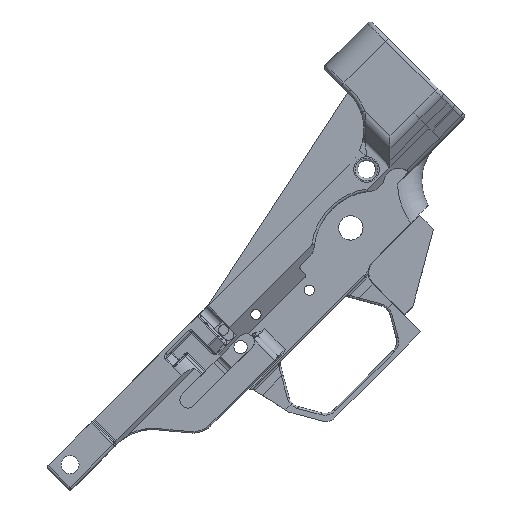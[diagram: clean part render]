
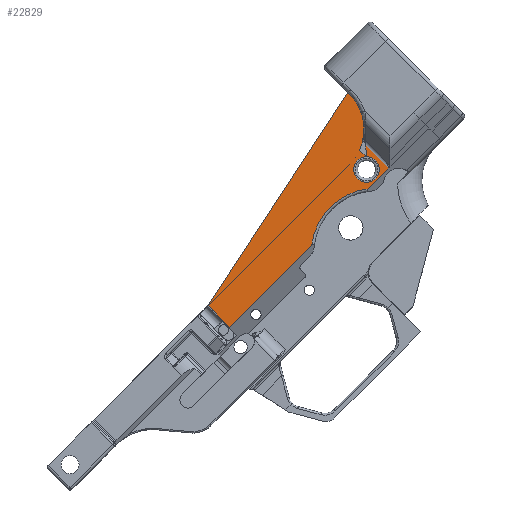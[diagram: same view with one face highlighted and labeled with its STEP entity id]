
A CAD part, front view. The second image highlights one B-rep face of the part: STEP entity #22829.
In plain terms, the highlighted planar face has unit normal (0, -1, 0).
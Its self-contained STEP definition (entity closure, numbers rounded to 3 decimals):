
#5562=CARTESIAN_POINT('',(-25.441,-18.567,22.339));
#5563=VERTEX_POINT('',#5562);
#5571=CARTESIAN_POINT('',(29.722,-18.567,77.502));
#5572=VERTEX_POINT('',#5571);
#5573=CARTESIAN_POINT('',(29.722,-18.567,77.502));
#5574=DIRECTION('',(-0.707,0.0,-0.707));
#5575=VECTOR('',#5574,78.013);
#5576=LINE('',#5573,#5575);
#5577=EDGE_CURVE('',#5572,#5563,#5576,.T.);
#9678=CARTESIAN_POINT('',(45.024,-18.567,76.019));
#9679=VERTEX_POINT('',#9678);
#9686=CARTESIAN_POINT('',(36.922,-18.567,67.916));
#9687=VERTEX_POINT('',#9686);
#9688=CARTESIAN_POINT('',(45.024,-18.567,76.019));
#9689=DIRECTION('',(-0.707,0.,-0.707));
#9690=VECTOR('',#9689,11.459);
#9691=LINE('',#9688,#9690);
#9692=EDGE_CURVE('',#9679,#9687,#9691,.T.);
#10764=CARTESIAN_POINT('',(41.289,-18.567,75.425));
#10765=VERTEX_POINT('',#10764);
#10766=CARTESIAN_POINT('',(36.289,-18.567,75.425));
#10767=DIRECTION('',(0.0,-1.0,0.0));
#10768=DIRECTION('',(1.0,0.0,0.0));
#10769=AXIS2_PLACEMENT_3D('',#10766,#10767,#10768);
#10770=CIRCLE('',#10769,5.);
#10771=EDGE_CURVE('',#10765,#10765,#10770,.T.);
#10781=CARTESIAN_POINT('',(29.013,-18.567,105.505));
#10782=VERTEX_POINT('',#10781);
#10783=CARTESIAN_POINT('',(35.207,-18.567,88.44));
#10784=VERTEX_POINT('',#10783);
#10785=CARTESIAN_POINT('',(16.079,-18.567,91.154));
#10786=DIRECTION('',(0.0,1.0,0.0));
#10787=DIRECTION('',(1.0,0.0,0.0));
#10788=AXIS2_PLACEMENT_3D('',#10785,#10786,#10787);
#10789=CIRCLE('',#10788,19.32);
#10790=EDGE_CURVE('',#10782,#10784,#10789,.T.);
#22725=CARTESIAN_POINT('',(-58.932,-18.567,-27.938));
#22726=DIRECTION('',(0.0,1.0,0.0));
#22727=DIRECTION('',(0.0,0.0,1.0));
#22728=AXIS2_PLACEMENT_3D('',#22725,#22726,#22727);
#22729=PLANE('',#22728);
#22730=ORIENTED_EDGE('',*,*,#9692,.F.);
#22731=CARTESIAN_POINT('',(35.986,-18.567,85.057));
#22732=VERTEX_POINT('',#22731);
#22733=CARTESIAN_POINT('',(45.024,-18.567,76.019));
#22734=DIRECTION('',(-0.707,0.0,0.707));
#22735=VECTOR('',#22734,12.782);
#22736=LINE('',#22733,#22735);
#22737=EDGE_CURVE('',#9679,#22732,#22736,.T.);
#22738=ORIENTED_EDGE('',*,*,#22737,.T.);
#22739=CARTESIAN_POINT('',(35.234,-18.567,87.194));
#22740=VERTEX_POINT('',#22739);
#22741=CARTESIAN_POINT('',(35.986,-18.567,85.057));
#22742=CARTESIAN_POINT('',(35.917,-18.567,85.232));
#22743=CARTESIAN_POINT('',(35.845,-18.566,85.408));
#22744=CARTESIAN_POINT('',(35.775,-18.566,85.583));
#22745=CARTESIAN_POINT('',(35.713,-18.566,85.735));
#22746=CARTESIAN_POINT('',(35.652,-18.567,85.886));
#22747=CARTESIAN_POINT('',(35.594,-18.567,86.04));
#22748=CARTESIAN_POINT('',(35.585,-18.567,86.063));
#22749=CARTESIAN_POINT('',(35.576,-18.567,86.087));
#22750=CARTESIAN_POINT('',(35.567,-18.567,86.11));
#22751=CARTESIAN_POINT('',(35.434,-18.567,86.464));
#22752=CARTESIAN_POINT('',(35.312,-18.567,86.821));
#22753=CARTESIAN_POINT('',(35.234,-18.567,87.194));
#22754=B_SPLINE_CURVE_WITH_KNOTS('',3,(#22741,#22742,#22743,#22744,#22745,#22746,#22747,#22748,#22749,#22750,#22751,#22752,#22753),.UNSPECIFIED.,.F.,.U.,(4,3,3,3,4),(-0.002,-0.002,-0.001,-0.001,0.0),.UNSPECIFIED.);
#22755=EDGE_CURVE('',#22732,#22740,#22754,.T.);
#22756=ORIENTED_EDGE('',*,*,#22755,.T.);
#22757=CARTESIAN_POINT('',(35.234,-18.567,87.194));
#22758=CARTESIAN_POINT('',(35.192,-18.567,87.398));
#22759=CARTESIAN_POINT('',(35.171,-18.567,87.608));
#22760=CARTESIAN_POINT('',(35.164,-18.567,88.024));
#22761=CARTESIAN_POINT('',(35.178,-18.567,88.234));
#22762=CARTESIAN_POINT('',(35.207,-18.567,88.44));
#22763=B_SPLINE_CURVE_WITH_KNOTS('',3,(#22757,#22758,#22759,#22760,#22761,#22762),.UNSPECIFIED.,.F.,.U.,(4,2,4),(-0.125,-0.062,0.),.UNSPECIFIED.);
#22764=EDGE_CURVE('',#22740,#10784,#22763,.T.);
#22765=ORIENTED_EDGE('',*,*,#22764,.T.);
#22766=ORIENTED_EDGE('',*,*,#10790,.F.);
#22767=CARTESIAN_POINT('',(29.722,-18.567,104.797));
#22768=VERTEX_POINT('',#22767);
#22769=CARTESIAN_POINT('',(29.013,-18.567,105.505));
#22770=DIRECTION('',(0.707,0.0,-0.707));
#22771=VECTOR('',#22770,1.002);
#22772=LINE('',#22769,#22771);
#22773=EDGE_CURVE('',#10782,#22768,#22772,.T.);
#22774=ORIENTED_EDGE('',*,*,#22773,.T.);
#22775=CARTESIAN_POINT('',(16.075,-18.567,91.15));
#22776=DIRECTION('',(0.0,-1.0,0.0));
#22777=DIRECTION('',(-1.0,0.0,0.0));
#22778=AXIS2_PLACEMENT_3D('',#22775,#22776,#22777);
#22779=CIRCLE('',#22778,19.3);
#22780=EDGE_CURVE('',#5572,#22768,#22779,.T.);
#22781=ORIENTED_EDGE('',*,*,#22780,.F.);
#22782=ORIENTED_EDGE('',*,*,#5577,.T.);
#22783=CARTESIAN_POINT('',(-23.477,-18.567,20.375));
#22784=VERTEX_POINT('',#22783);
#22785=CARTESIAN_POINT('',(-23.477,-18.567,20.375));
#22786=DIRECTION('',(-0.707,0.0,0.707));
#22787=VECTOR('',#22786,2.778);
#22788=LINE('',#22785,#22787);
#22789=EDGE_CURVE('',#22784,#5563,#22788,.T.);
#22790=ORIENTED_EDGE('',*,*,#22789,.F.);
#22791=CARTESIAN_POINT('',(-23.502,-18.566,20.35));
#22792=VERTEX_POINT('',#22791);
#22793=CARTESIAN_POINT('',(-23.502,-18.566,20.35));
#22794=CARTESIAN_POINT('',(-23.493,-18.566,20.358));
#22795=CARTESIAN_POINT('',(-23.485,-18.567,20.367));
#22796=CARTESIAN_POINT('',(-23.477,-18.567,20.375));
#22797=B_SPLINE_CURVE_WITH_KNOTS('',3,(#22793,#22794,#22795,#22796),.UNSPECIFIED.,.F.,.U.,(4,4),(0.001,1.0),.UNSPECIFIED.);
#22798=EDGE_CURVE('',#22792,#22784,#22797,.T.);
#22799=ORIENTED_EDGE('',*,*,#22798,.F.);
#22800=CARTESIAN_POINT('',(-17.081,-18.567,13.914));
#22801=VERTEX_POINT('',#22800);
#22802=CARTESIAN_POINT('',(-17.081,-18.567,13.914));
#22803=CARTESIAN_POINT('',(-19.221,-18.567,16.059));
#22804=CARTESIAN_POINT('',(-21.361,-18.567,18.205));
#22805=CARTESIAN_POINT('',(-23.502,-18.567,20.35));
#22806=QUASI_UNIFORM_CURVE('',3,(#22802,#22803,#22804,#22805),.UNSPECIFIED.,.F.,.U.);
#22807=EDGE_CURVE('',#22801,#22792,#22806,.T.);
#22808=ORIENTED_EDGE('',*,*,#22807,.F.);
#22809=CARTESIAN_POINT('',(14.954,-18.567,45.948));
#22810=VERTEX_POINT('',#22809);
#22811=CARTESIAN_POINT('',(14.954,-18.567,45.948));
#22812=DIRECTION('',(-0.707,0.,-0.707));
#22813=VECTOR('',#22812,45.303);
#22814=LINE('',#22811,#22813);
#22815=EDGE_CURVE('',#22810,#22801,#22814,.T.);
#22816=ORIENTED_EDGE('',*,*,#22815,.F.);
#22817=CARTESIAN_POINT('',(40.004,-18.567,42.866));
#22818=DIRECTION('',(0.,-1.0,0.));
#22819=DIRECTION('',(-0.993,0.,0.122));
#22820=AXIS2_PLACEMENT_3D('',#22817,#22818,#22819);
#22821=CIRCLE('',#22820,25.239);
#22822=EDGE_CURVE('',#9687,#22810,#22821,.T.);
#22823=ORIENTED_EDGE('',*,*,#22822,.F.);
#22824=EDGE_LOOP('',(#22730,#22738,#22756,#22765,#22766,#22774,#22781,#22782,#22790,#22799,#22808,#22816,#22823));
#22825=FACE_OUTER_BOUND('',#22824,.T.);
#22826=ORIENTED_EDGE('',*,*,#10771,.F.);
#22827=EDGE_LOOP('',(#22826));
#22828=FACE_BOUND('',#22827,.T.);
#22829=ADVANCED_FACE('',(#22825,#22828),#22729,.F.);
